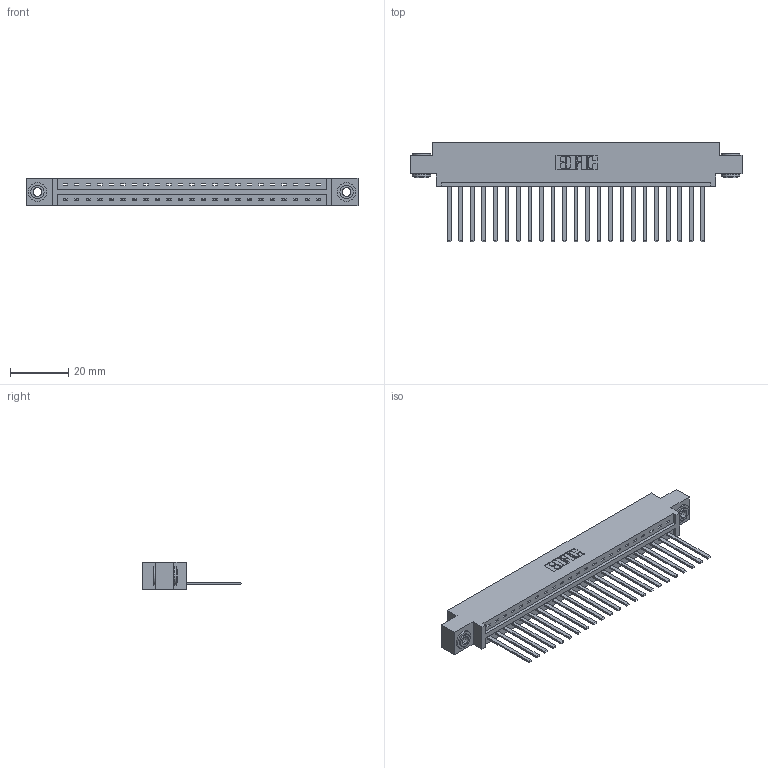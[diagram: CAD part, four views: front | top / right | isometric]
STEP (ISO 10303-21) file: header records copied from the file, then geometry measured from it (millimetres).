
FILE_DESCRIPTION (( 'STEP AP203' ), '1' );
FILE_NAME ('337-023-544-603.STEP', '2018-08-05T17:30:21', ( '' ), ( '' ), 'SwSTEP 2.0', 'SolidWorks 2016', '' );
FILE_SCHEMA (( 'CONFIG_CONTROL_DESIGN' ));
Length unit declared in the file: inch
Products named in the file (4): 345-250-002_345-250-002-102; 337-023-544-603; 337 Part_0.170 Offset - 0.156 Dia-TH; 345-292-001_345-293-144
Assembly tree (26 placements, depth 2):
  337-023-544-603
    337 Part_0.170 Offset - 0.156 Dia-TH
    345-292-001_345-293-144  x23
    345-250-002_345-250-002-102  x2
Bounding box: 114.15 x 34.3 x 9.4 mm (x, y, z)
Volume: 11794.2 mm3; surface area: 13287.5 mm2
Topology: 26 solids, 26 shells, 1444 faces, 4309 edges, 2838 vertices
Faces by surface type: plane 1050, cylinder 386, cone 8
Entity records: 20152 total; most frequent: CARTESIAN_POINT 3486, ORIENTED_EDGE 3438, DIRECTION 3003, EDGE_CURVE 1719, LINE 1571, VECTOR 1571, VERTEX_POINT 1142, AXIS2_PLACEMENT_3D 716
